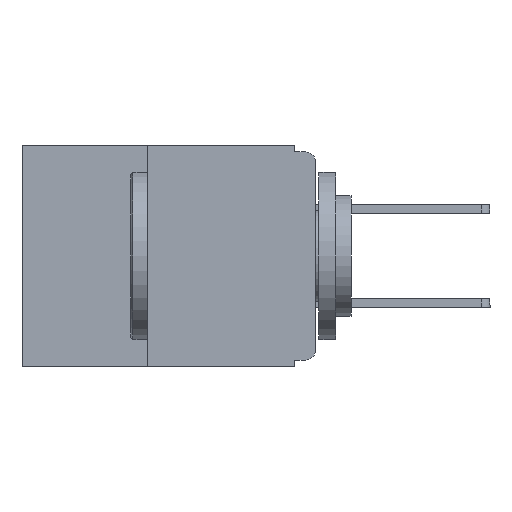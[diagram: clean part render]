
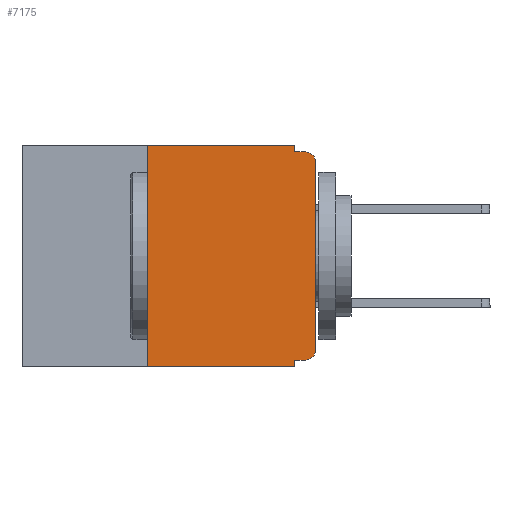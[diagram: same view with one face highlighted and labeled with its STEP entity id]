
A CAD part, left-side view. The second image highlights one B-rep face of the part: STEP entity #7175.
In plain terms, the highlighted planar face has unit normal (-1, 0, 0).
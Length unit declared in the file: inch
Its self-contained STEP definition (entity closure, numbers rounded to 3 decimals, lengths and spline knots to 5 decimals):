
#221 = CARTESIAN_POINT ( 'NONE',  ( 0., 0., -0.305 ) ) ;
#628 = VERTEX_POINT ( 'NONE', #1911 ) ;
#838 = ORIENTED_EDGE ( 'NONE', *, *, #2250, .F. ) ;
#933 = LINE ( 'NONE', #17426, #16244 ) ;
#939 = CARTESIAN_POINT ( 'NONE',  ( 0., 0.031, 0. ) ) ;
#1128 = DIRECTION ( 'NONE',  ( 0., -1., 0. ) ) ;
#1337 = CARTESIAN_POINT ( 'NONE',  ( 0., 0., 0. ) ) ;
#1395 = VECTOR ( 'NONE', #11626, 39.37008 ) ;
#1509 = VERTEX_POINT ( 'NONE', #17396 ) ;
#1911 = CARTESIAN_POINT ( 'NONE',  ( 0., 0.015, -0.32 ) ) ;
#2047 = LINE ( 'NONE', #1337, #8754 ) ;
#2250 = EDGE_CURVE ( 'NONE', #8049, #7635, #5206, .T. ) ;
#2326 = AXIS2_PLACEMENT_3D ( 'NONE', #8292, #8179, #8076 ) ;
#2714 = EDGE_CURVE ( 'NONE', #17978, #12735, #933, .T. ) ;
#2785 = LINE ( 'NONE', #18321, #9984 ) ;
#3020 = CARTESIAN_POINT ( 'NONE',  ( 0., 0.25, -0.33 ) ) ;
#3191 = EDGE_CURVE ( 'NONE', #17642, #12422, #10272, .T. ) ;
#3948 = CARTESIAN_POINT ( 'NONE',  ( 0., 0.015, -0.305 ) ) ;
#3952 = ORIENTED_EDGE ( 'NONE', *, *, #15602, .F. ) ;
#4275 = CARTESIAN_POINT ( 'NONE',  ( 0., 0.031, -0.01 ) ) ;
#4376 = VECTOR ( 'NONE', #9519, 39.37008 ) ;
#4445 = EDGE_LOOP ( 'NONE', ( #14577, #7777, #16347, #16578, #3952, #16818, #18125, #838, #8875, #5982 ) ) ;
#4655 = VERTEX_POINT ( 'NONE', #9363 ) ;
#4796 = CARTESIAN_POINT ( 'NONE',  ( 0., 0.031, -0.33 ) ) ;
#4828 = LINE ( 'NONE', #16741, #4376 ) ;
#4973 = VECTOR ( 'NONE', #8714, 39.37008 ) ;
#5083 = CARTESIAN_POINT ( 'NONE',  ( 0., 0.031, -0.32 ) ) ;
#5206 = LINE ( 'NONE', #9658, #1395 ) ;
#5394 = DIRECTION ( 'NONE',  ( 0., 0., -1. ) ) ;
#5982 = ORIENTED_EDGE ( 'NONE', *, *, #15588, .T. ) ;
#6238 = CARTESIAN_POINT ( 'NONE',  ( 0., 0., -0.32 ) ) ;
#6517 = VECTOR ( 'NONE', #12652, 39.37008 ) ;
#7175 = ADVANCED_FACE ( 'NONE', ( #12187 ), #15214, .F. ) ;
#7635 = VERTEX_POINT ( 'NONE', #4796 ) ;
#7777 = ORIENTED_EDGE ( 'NONE', *, *, #3191, .T. ) ;
#7979 = CARTESIAN_POINT ( 'NONE',  ( 0., 0.015, -0.01 ) ) ;
#8049 = VERTEX_POINT ( 'NONE', #5083 ) ;
#8076 = DIRECTION ( 'NONE',  ( 0., 0., -1. ) ) ;
#8179 = DIRECTION ( 'NONE',  ( -1., 0., 0. ) ) ;
#8200 = VERTEX_POINT ( 'NONE', #221 ) ;
#8292 = CARTESIAN_POINT ( 'NONE',  ( 0., 0.015, -0.025 ) ) ;
#8522 = CARTESIAN_POINT ( 'NONE',  ( 0., 0., -0.025 ) ) ;
#8523 = EDGE_CURVE ( 'NONE', #4655, #7635, #10317, .T. ) ;
#8714 = DIRECTION ( 'NONE',  ( 0., 0., 1. ) ) ;
#8754 = VECTOR ( 'NONE', #14270, 39.37008 ) ;
#8875 = ORIENTED_EDGE ( 'NONE', *, *, #14802, .F. ) ;
#9363 = CARTESIAN_POINT ( 'NONE',  ( 0., 0.25, -0.33 ) ) ;
#9519 = DIRECTION ( 'NONE',  ( 0., -1., 0. ) ) ;
#9658 = CARTESIAN_POINT ( 'NONE',  ( 0., 0.031, -0.33 ) ) ;
#9984 = VECTOR ( 'NONE', #1128, 39.37008 ) ;
#10272 = CIRCLE ( 'NONE', #2326, 0.015 ) ;
#10317 = LINE ( 'NONE', #12915, #6517 ) ;
#10426 = EDGE_CURVE ( 'NONE', #12735, #12422, #4828, .T. ) ;
#10429 = CIRCLE ( 'NONE', #12551, 0.015 ) ;
#11626 = DIRECTION ( 'NONE',  ( 0., 0., -1. ) ) ;
#12025 = DIRECTION ( 'NONE',  ( 0., 1., 0. ) ) ;
#12113 = DIRECTION ( 'NONE',  ( 0., 0., -1. ) ) ;
#12187 = FACE_OUTER_BOUND ( 'NONE', #4445, .T. ) ;
#12365 = VECTOR ( 'NONE', #12025, 39.37008 ) ;
#12422 = VERTEX_POINT ( 'NONE', #7979 ) ;
#12551 = AXIS2_PLACEMENT_3D ( 'NONE', #3948, #14072, #5394 ) ;
#12652 = DIRECTION ( 'NONE',  ( 0., -1., 0. ) ) ;
#12735 = VERTEX_POINT ( 'NONE', #4275 ) ;
#12915 = CARTESIAN_POINT ( 'NONE',  ( 0., 0.437, -0.33 ) ) ;
#13314 = EDGE_CURVE ( 'NONE', #8200, #17642, #2047, .T. ) ;
#14072 = DIRECTION ( 'NONE',  ( -1., 0., 0. ) ) ;
#14112 = AXIS2_PLACEMENT_3D ( 'NONE', #16119, #14719, #14194 ) ;
#14194 = DIRECTION ( 'NONE',  ( 0., 0., -1. ) ) ;
#14270 = DIRECTION ( 'NONE',  ( 0., 0., 1. ) ) ;
#14577 = ORIENTED_EDGE ( 'NONE', *, *, #13314, .T. ) ;
#14719 = DIRECTION ( 'NONE',  ( 1., 0., 0. ) ) ;
#14802 = EDGE_CURVE ( 'NONE', #628, #8049, #16221, .T. ) ;
#15214 = PLANE ( 'NONE',  #14112 ) ;
#15588 = EDGE_CURVE ( 'NONE', #628, #8200, #10429, .T. ) ;
#15602 = EDGE_CURVE ( 'NONE', #1509, #17978, #2785, .T. ) ;
#16119 = CARTESIAN_POINT ( 'NONE',  ( 0., 0.437, 0. ) ) ;
#16221 = LINE ( 'NONE', #6238, #12365 ) ;
#16244 = VECTOR ( 'NONE', #12113, 39.37008 ) ;
#16347 = ORIENTED_EDGE ( 'NONE', *, *, #10426, .F. ) ;
#16481 = LINE ( 'NONE', #3020, #4973 ) ;
#16578 = ORIENTED_EDGE ( 'NONE', *, *, #2714, .F. ) ;
#16741 = CARTESIAN_POINT ( 'NONE',  ( 0., 0., -0.01 ) ) ;
#16818 = ORIENTED_EDGE ( 'NONE', *, *, #17105, .F. ) ;
#17105 = EDGE_CURVE ( 'NONE', #4655, #1509, #16481, .T. ) ;
#17396 = CARTESIAN_POINT ( 'NONE',  ( 0., 0.25, 0. ) ) ;
#17426 = CARTESIAN_POINT ( 'NONE',  ( 0., 0.031, 0. ) ) ;
#17642 = VERTEX_POINT ( 'NONE', #8522 ) ;
#17978 = VERTEX_POINT ( 'NONE', #939 ) ;
#18125 = ORIENTED_EDGE ( 'NONE', *, *, #8523, .T. ) ;
#18321 = CARTESIAN_POINT ( 'NONE',  ( 0., 0.437, 0. ) ) ;
